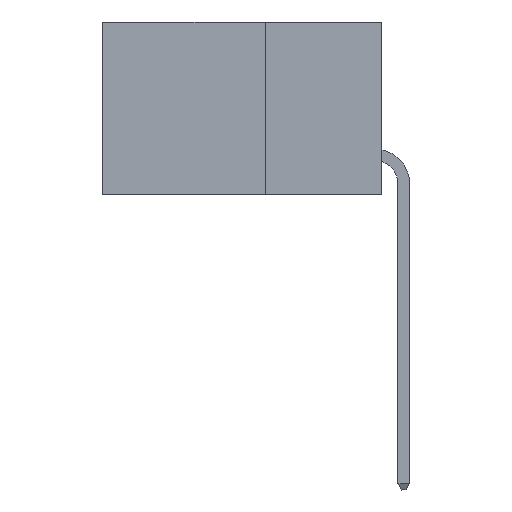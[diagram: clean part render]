
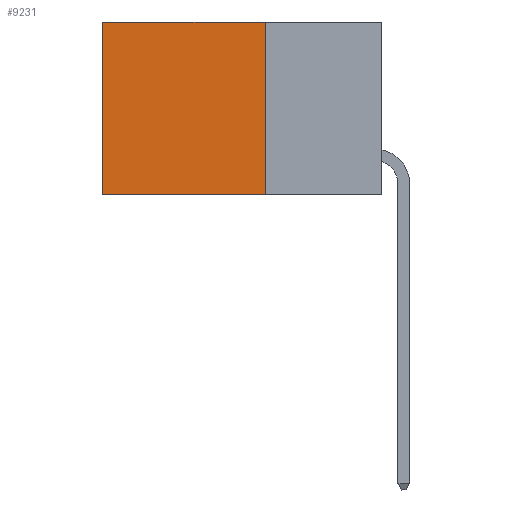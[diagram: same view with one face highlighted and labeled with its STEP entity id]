
A CAD part, left-side view. The second image highlights one B-rep face of the part: STEP entity #9231.
In plain terms, the highlighted planar face has unit normal (-1, 0, 0).
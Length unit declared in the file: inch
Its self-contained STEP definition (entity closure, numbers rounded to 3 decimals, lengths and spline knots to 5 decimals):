
#218 = CARTESIAN_POINT ( 'NONE',  ( 0.2875, 0.6, 0. ) ) ;
#635 = CARTESIAN_POINT ( 'NONE',  ( 0.2875, 0.6, 0. ) ) ;
#1238 = EDGE_CURVE ( 'NONE', #11397, #9896, #10703, .T. ) ;
#1641 = CARTESIAN_POINT ( 'NONE',  ( 0.2875, 0.25, -0.37 ) ) ;
#1644 = VECTOR ( 'NONE', #9492, 39.37008 ) ;
#1661 = DIRECTION ( 'NONE',  ( 1., 0., 0. ) ) ;
#2732 = EDGE_CURVE ( 'NONE', #9896, #10245, #11150, .T. ) ;
#3285 = CARTESIAN_POINT ( 'NONE',  ( 0.2875, 0.25, 0. ) ) ;
#3330 = DIRECTION ( 'NONE',  ( 0., 0., -1. ) ) ;
#3907 = LINE ( 'NONE', #635, #9905 ) ;
#4436 = ORIENTED_EDGE ( 'NONE', *, *, #7097, .T. ) ;
#4558 = ORIENTED_EDGE ( 'NONE', *, *, #2732, .F. ) ;
#4657 = ORIENTED_EDGE ( 'NONE', *, *, #1238, .F. ) ;
#4715 = ORIENTED_EDGE ( 'NONE', *, *, #5772, .T. ) ;
#4899 = FACE_OUTER_BOUND ( 'NONE', #5076, .T. ) ;
#4975 = VERTEX_POINT ( 'NONE', #218 ) ;
#5076 = EDGE_LOOP ( 'NONE', ( #4436, #4558, #4657, #4715 ) ) ;
#5772 = EDGE_CURVE ( 'NONE', #11397, #4975, #11252, .T. ) ;
#6113 = PLANE ( 'NONE',  #14234 ) ;
#6215 = CARTESIAN_POINT ( 'NONE',  ( 0.2875, 0.25, 0. ) ) ;
#7097 = EDGE_CURVE ( 'NONE', #4975, #10245, #3907, .T. ) ;
#7397 = VECTOR ( 'NONE', #3330, 39.37008 ) ;
#8362 = CARTESIAN_POINT ( 'NONE',  ( 0.2875, 0.25, 0. ) ) ;
#9014 = CARTESIAN_POINT ( 'NONE',  ( 0.2875, 0.6, -0.37 ) ) ;
#9231 = ADVANCED_FACE ( 'NONE', ( #4899 ), #6113, .F. ) ;
#9492 = DIRECTION ( 'NONE',  ( 0., 1., 0. ) ) ;
#9503 = DIRECTION ( 'NONE',  ( 0., 0., -1. ) ) ;
#9614 = DIRECTION ( 'NONE',  ( 0., 0., -1. ) ) ;
#9896 = VERTEX_POINT ( 'NONE', #1641 ) ;
#9905 = VECTOR ( 'NONE', #9614, 39.37008 ) ;
#10245 = VERTEX_POINT ( 'NONE', #9014 ) ;
#10495 = CARTESIAN_POINT ( 'NONE',  ( 0.2875, 0.25, -0.37 ) ) ;
#10566 = CARTESIAN_POINT ( 'NONE',  ( 0.2875, 0.25, 0. ) ) ;
#10636 = DIRECTION ( 'NONE',  ( 0., 1., 0. ) ) ;
#10703 = LINE ( 'NONE', #3285, #7397 ) ;
#11150 = LINE ( 'NONE', #10495, #13707 ) ;
#11252 = LINE ( 'NONE', #10566, #1644 ) ;
#11397 = VERTEX_POINT ( 'NONE', #6215 ) ;
#13707 = VECTOR ( 'NONE', #10636, 39.37008 ) ;
#14234 = AXIS2_PLACEMENT_3D ( 'NONE', #8362, #1661, #9503 ) ;
